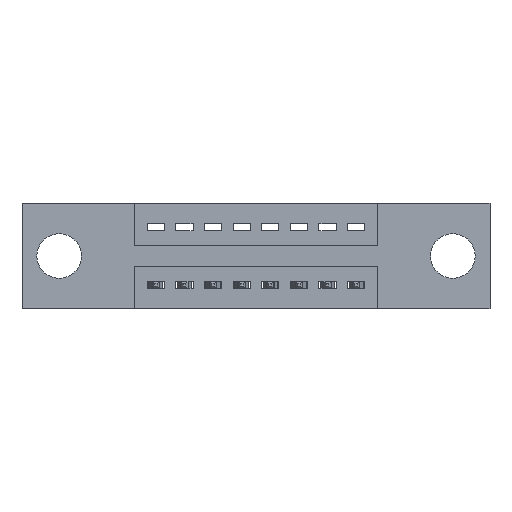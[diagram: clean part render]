
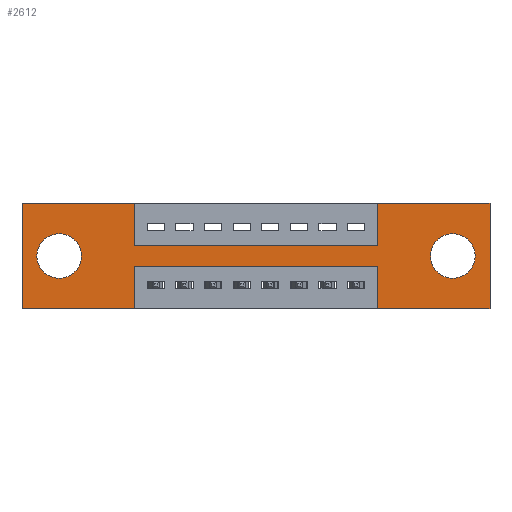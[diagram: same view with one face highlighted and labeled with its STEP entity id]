
A CAD part, front view. The second image highlights one B-rep face of the part: STEP entity #2612.
In plain terms, the highlighted planar face has unit normal (0, -1, 0).
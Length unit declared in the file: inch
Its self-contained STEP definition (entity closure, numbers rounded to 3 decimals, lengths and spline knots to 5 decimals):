
#33 = CIRCLE ( 'NONE', #931, 0.078 ) ;
#421 = CARTESIAN_POINT ( 'NONE',  ( 0., 0., -0.37 ) ) ;
#510 = LINE ( 'NONE', #3244, #4498 ) ;
#668 = VECTOR ( 'NONE', #10567, 39.37008 ) ;
#713 = LINE ( 'NONE', #9267, #3044 ) ;
#725 = ORIENTED_EDGE ( 'NONE', *, *, #7087, .F. ) ;
#789 = CARTESIAN_POINT ( 'NONE',  ( 0.3925, 0., 0. ) ) ;
#817 = ORIENTED_EDGE ( 'NONE', *, *, #3673, .F. ) ;
#821 = EDGE_CURVE ( 'NONE', #10786, #3272, #7708, .T. ) ;
#828 = LINE ( 'NONE', #10262, #5307 ) ;
#898 = VERTEX_POINT ( 'NONE', #4633 ) ;
#913 = ORIENTED_EDGE ( 'NONE', *, *, #8810, .T. ) ;
#931 = AXIS2_PLACEMENT_3D ( 'NONE', #10570, #5396, #7906 ) ;
#1103 = AXIS2_PLACEMENT_3D ( 'NONE', #4903, #2219, #1590 ) ;
#1408 = AXIS2_PLACEMENT_3D ( 'NONE', #8926, #4566, #4732 ) ;
#1479 = VECTOR ( 'NONE', #9799, 39.37008 ) ;
#1513 = CARTESIAN_POINT ( 'NONE',  ( 1.635, 0., -0.37 ) ) ;
#1590 = DIRECTION ( 'NONE',  ( 0., 0., 1. ) ) ;
#1737 = CARTESIAN_POINT ( 'NONE',  ( 1.505, 0., -0.107 ) ) ;
#1766 = EDGE_CURVE ( 'NONE', #3272, #3820, #3864, .T. ) ;
#1815 = VERTEX_POINT ( 'NONE', #3192 ) ;
#1817 = DIRECTION ( 'NONE',  ( 0., 1., 0. ) ) ;
#1904 = VERTEX_POINT ( 'NONE', #1513 ) ;
#2077 = CARTESIAN_POINT ( 'NONE',  ( 0., 0., 0. ) ) ;
#2219 = DIRECTION ( 'NONE',  ( 0., 1., 0. ) ) ;
#2612 = ADVANCED_FACE ( 'NONE', ( #6236, #5407, #6292 ), #9692, .T. ) ;
#2731 = VERTEX_POINT ( 'NONE', #4216 ) ;
#2948 = EDGE_LOOP ( 'NONE', ( #4768, #4754 ) ) ;
#3004 = ORIENTED_EDGE ( 'NONE', *, *, #10552, .F. ) ;
#3044 = VECTOR ( 'NONE', #7649, 39.37008 ) ;
#3056 = CARTESIAN_POINT ( 'NONE',  ( 0., 0., 0. ) ) ;
#3157 = ORIENTED_EDGE ( 'NONE', *, *, #821, .F. ) ;
#3192 = CARTESIAN_POINT ( 'NONE',  ( 0.13, 0., -0.263 ) ) ;
#3241 = VERTEX_POINT ( 'NONE', #1737 ) ;
#3244 = CARTESIAN_POINT ( 'NONE',  ( 0., 0., -0.37 ) ) ;
#3272 = VERTEX_POINT ( 'NONE', #789 ) ;
#3279 = CARTESIAN_POINT ( 'NONE',  ( 1.2425, 0., -0.22 ) ) ;
#3419 = VERTEX_POINT ( 'NONE', #8106 ) ;
#3477 = EDGE_CURVE ( 'NONE', #7923, #7081, #5432, .T. ) ;
#3673 = EDGE_CURVE ( 'NONE', #5260, #7923, #828, .T. ) ;
#3686 = DIRECTION ( 'NONE',  ( -1., 0., 0. ) ) ;
#3709 = LINE ( 'NONE', #3769, #1479 ) ;
#3757 = CARTESIAN_POINT ( 'NONE',  ( 0.3925, 0., 0. ) ) ;
#3769 = CARTESIAN_POINT ( 'NONE',  ( 0., 0., -0.37 ) ) ;
#3820 = VERTEX_POINT ( 'NONE', #7040 ) ;
#3864 = LINE ( 'NONE', #3757, #668 ) ;
#3932 = VERTEX_POINT ( 'NONE', #9705 ) ;
#3939 = DIRECTION ( 'NONE',  ( 0., 0., -1. ) ) ;
#4016 = ORIENTED_EDGE ( 'NONE', *, *, #5024, .T. ) ;
#4159 = LINE ( 'NONE', #9855, #10581 ) ;
#4216 = CARTESIAN_POINT ( 'NONE',  ( 0.13, 0., -0.107 ) ) ;
#4219 = DIRECTION ( 'NONE',  ( 1., 0., 0. ) ) ;
#4288 = VECTOR ( 'NONE', #10175, 39.37008 ) ;
#4326 = EDGE_LOOP ( 'NONE', ( #6645, #6560, #817, #9793, #3004, #7979, #5738, #5196, #9281, #3157, #725, #7047 ) ) ;
#4429 = VERTEX_POINT ( 'NONE', #9741 ) ;
#4485 = CARTESIAN_POINT ( 'NONE',  ( 0.3925, 0., -0.37 ) ) ;
#4498 = VECTOR ( 'NONE', #7552, 39.37008 ) ;
#4518 = VERTEX_POINT ( 'NONE', #4485 ) ;
#4566 = DIRECTION ( 'NONE',  ( 0., 1., 0. ) ) ;
#4633 = CARTESIAN_POINT ( 'NONE',  ( 0., 0., -0.37 ) ) ;
#4649 = CARTESIAN_POINT ( 'NONE',  ( 0.3925, 0., -0.22 ) ) ;
#4687 = CARTESIAN_POINT ( 'NONE',  ( 1.505, 0., -0.263 ) ) ;
#4732 = DIRECTION ( 'NONE',  ( 0., 0., 1. ) ) ;
#4754 = ORIENTED_EDGE ( 'NONE', *, *, #8959, .T. ) ;
#4768 = ORIENTED_EDGE ( 'NONE', *, *, #5479, .T. ) ;
#4903 = CARTESIAN_POINT ( 'NONE',  ( 0.13, 0., -0.185 ) ) ;
#5024 = EDGE_CURVE ( 'NONE', #2731, #1815, #8554, .T. ) ;
#5181 = CARTESIAN_POINT ( 'NONE',  ( 0.3925, 0., -0.15 ) ) ;
#5196 = ORIENTED_EDGE ( 'NONE', *, *, #6690, .F. ) ;
#5260 = VERTEX_POINT ( 'NONE', #8192 ) ;
#5270 = LINE ( 'NONE', #10226, #4288 ) ;
#5307 = VECTOR ( 'NONE', #5985, 39.37008 ) ;
#5344 = LINE ( 'NONE', #5181, #10884 ) ;
#5396 = DIRECTION ( 'NONE',  ( 0., 1., 0. ) ) ;
#5407 = FACE_BOUND ( 'NONE', #10842, .T. ) ;
#5432 = LINE ( 'NONE', #4649, #9225 ) ;
#5479 = EDGE_CURVE ( 'NONE', #3241, #9984, #33, .T. ) ;
#5622 = DIRECTION ( 'NONE',  ( 0., 0., -1. ) ) ;
#5738 = ORIENTED_EDGE ( 'NONE', *, *, #7646, .F. ) ;
#5985 = DIRECTION ( 'NONE',  ( 0., 0., 1. ) ) ;
#6092 = DIRECTION ( 'NONE',  ( 1., 0., 0. ) ) ;
#6236 = FACE_BOUND ( 'NONE', #2948, .T. ) ;
#6292 = FACE_OUTER_BOUND ( 'NONE', #4326, .T. ) ;
#6359 = LINE ( 'NONE', #3056, #10400 ) ;
#6560 = ORIENTED_EDGE ( 'NONE', *, *, #3477, .F. ) ;
#6645 = ORIENTED_EDGE ( 'NONE', *, *, #7958, .F. ) ;
#6690 = EDGE_CURVE ( 'NONE', #3820, #4429, #5344, .T. ) ;
#6782 = CARTESIAN_POINT ( 'NONE',  ( 0.3925, 0., -0.22 ) ) ;
#6818 = CIRCLE ( 'NONE', #8244, 0.078 ) ;
#6928 = AXIS2_PLACEMENT_3D ( 'NONE', #421, #8029, #3939 ) ;
#6989 = LINE ( 'NONE', #10432, #7159 ) ;
#7040 = CARTESIAN_POINT ( 'NONE',  ( 0.3925, 0., -0.15 ) ) ;
#7045 = DIRECTION ( 'NONE',  ( 0., 0., 1. ) ) ;
#7047 = ORIENTED_EDGE ( 'NONE', *, *, #10393, .F. ) ;
#7081 = VERTEX_POINT ( 'NONE', #6782 ) ;
#7087 = EDGE_CURVE ( 'NONE', #898, #10786, #5270, .T. ) ;
#7159 = VECTOR ( 'NONE', #7045, 39.37008 ) ;
#7350 = CIRCLE ( 'NONE', #1103, 0.078 ) ;
#7552 = DIRECTION ( 'NONE',  ( -1., 0., 0. ) ) ;
#7646 = EDGE_CURVE ( 'NONE', #4429, #3932, #6989, .T. ) ;
#7649 = DIRECTION ( 'NONE',  ( 0., 0., -1. ) ) ;
#7708 = LINE ( 'NONE', #8770, #10636 ) ;
#7906 = DIRECTION ( 'NONE',  ( 0., 0., -1. ) ) ;
#7923 = VERTEX_POINT ( 'NONE', #3279 ) ;
#7958 = EDGE_CURVE ( 'NONE', #7081, #4518, #713, .T. ) ;
#7979 = ORIENTED_EDGE ( 'NONE', *, *, #9967, .F. ) ;
#8029 = DIRECTION ( 'NONE',  ( 0., -1., 0. ) ) ;
#8038 = DIRECTION ( 'NONE',  ( 1., 0., 0. ) ) ;
#8106 = CARTESIAN_POINT ( 'NONE',  ( 1.635, 0., 0. ) ) ;
#8192 = CARTESIAN_POINT ( 'NONE',  ( 1.2425, 0., -0.37 ) ) ;
#8244 = AXIS2_PLACEMENT_3D ( 'NONE', #10973, #1817, #11031 ) ;
#8554 = CIRCLE ( 'NONE', #1408, 0.078 ) ;
#8583 = EDGE_CURVE ( 'NONE', #1904, #5260, #510, .T. ) ;
#8770 = CARTESIAN_POINT ( 'NONE',  ( 0., 0., 0. ) ) ;
#8810 = EDGE_CURVE ( 'NONE', #1815, #2731, #7350, .T. ) ;
#8926 = CARTESIAN_POINT ( 'NONE',  ( 0.13, 0., -0.185 ) ) ;
#8959 = EDGE_CURVE ( 'NONE', #9984, #3241, #6818, .T. ) ;
#9225 = VECTOR ( 'NONE', #3686, 39.37008 ) ;
#9267 = CARTESIAN_POINT ( 'NONE',  ( 0.3925, 0., -0.37 ) ) ;
#9281 = ORIENTED_EDGE ( 'NONE', *, *, #1766, .F. ) ;
#9692 = PLANE ( 'NONE',  #6928 ) ;
#9705 = CARTESIAN_POINT ( 'NONE',  ( 1.2425, 0., 0. ) ) ;
#9741 = CARTESIAN_POINT ( 'NONE',  ( 1.2425, 0., -0.15 ) ) ;
#9793 = ORIENTED_EDGE ( 'NONE', *, *, #8583, .F. ) ;
#9799 = DIRECTION ( 'NONE',  ( -1., 0., 0. ) ) ;
#9855 = CARTESIAN_POINT ( 'NONE',  ( 1.635, 0., 0. ) ) ;
#9967 = EDGE_CURVE ( 'NONE', #3932, #3419, #6359, .T. ) ;
#9984 = VERTEX_POINT ( 'NONE', #4687 ) ;
#10175 = DIRECTION ( 'NONE',  ( 0., 0., 1. ) ) ;
#10226 = CARTESIAN_POINT ( 'NONE',  ( 0., 0., 0. ) ) ;
#10262 = CARTESIAN_POINT ( 'NONE',  ( 1.2425, 0., -0.37 ) ) ;
#10393 = EDGE_CURVE ( 'NONE', #4518, #898, #3709, .T. ) ;
#10400 = VECTOR ( 'NONE', #8038, 39.37008 ) ;
#10432 = CARTESIAN_POINT ( 'NONE',  ( 1.2425, 0., 0. ) ) ;
#10552 = EDGE_CURVE ( 'NONE', #3419, #1904, #4159, .T. ) ;
#10567 = DIRECTION ( 'NONE',  ( 0., 0., -1. ) ) ;
#10570 = CARTESIAN_POINT ( 'NONE',  ( 1.505, 0., -0.185 ) ) ;
#10581 = VECTOR ( 'NONE', #5622, 39.37008 ) ;
#10636 = VECTOR ( 'NONE', #6092, 39.37008 ) ;
#10786 = VERTEX_POINT ( 'NONE', #2077 ) ;
#10842 = EDGE_LOOP ( 'NONE', ( #4016, #913 ) ) ;
#10884 = VECTOR ( 'NONE', #4219, 39.37008 ) ;
#10973 = CARTESIAN_POINT ( 'NONE',  ( 1.505, 0., -0.185 ) ) ;
#11031 = DIRECTION ( 'NONE',  ( 0., 0., -1. ) ) ;
